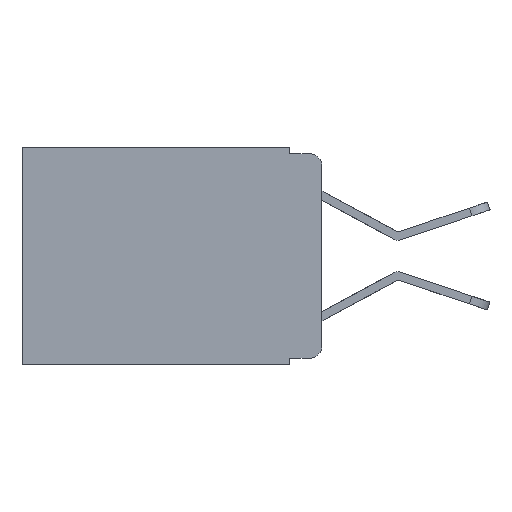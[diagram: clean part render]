
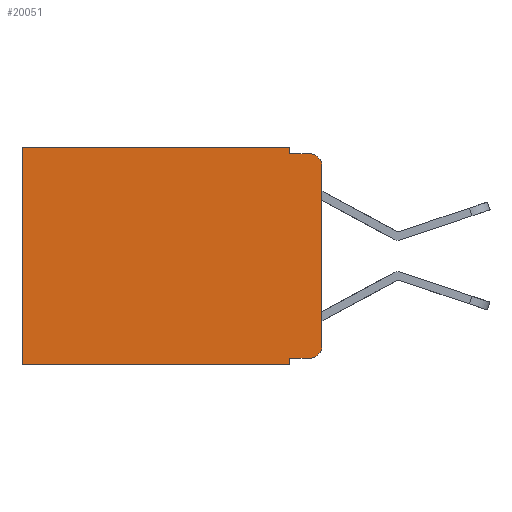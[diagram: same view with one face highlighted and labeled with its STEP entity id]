
A CAD part, left-side view. The second image highlights one B-rep face of the part: STEP entity #20051.
In plain terms, the highlighted planar face has unit normal (-1, 0, 0).
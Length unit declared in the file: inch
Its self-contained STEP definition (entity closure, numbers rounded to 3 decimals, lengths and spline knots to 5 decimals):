
#36 = EDGE_CURVE ( 'NONE', #19604, #1317, #16578, .T. ) ;
#1054 = ORIENTED_EDGE ( 'NONE', *, *, #10838, .F. ) ;
#1122 = DIRECTION ( 'NONE',  ( 0., -1., 0. ) ) ;
#1317 = VERTEX_POINT ( 'NONE', #21153 ) ;
#1393 = DIRECTION ( 'NONE',  ( 0., -1., 0. ) ) ;
#1402 = CARTESIAN_POINT ( 'NONE',  ( 0.298, 0.051, 0. ) ) ;
#1448 = EDGE_CURVE ( 'NONE', #19604, #22736, #23890, .T. ) ;
#1481 = CARTESIAN_POINT ( 'NONE',  ( 0.298, 0., -0.313 ) ) ;
#1501 = LINE ( 'NONE', #11058, #10415 ) ;
#1670 = DIRECTION ( 'NONE',  ( 0., 0., -1. ) ) ;
#1957 = CARTESIAN_POINT ( 'NONE',  ( 0.298, 0.051, -0.01 ) ) ;
#2050 = CARTESIAN_POINT ( 'NONE',  ( 0.298, 0.02, -0.313 ) ) ;
#2100 = AXIS2_PLACEMENT_3D ( 'NONE', #2050, #15978, #4168 ) ;
#2465 = LINE ( 'NONE', #7509, #22039 ) ;
#2858 = EDGE_CURVE ( 'NONE', #3120, #16821, #24452, .T. ) ;
#3104 = CARTESIAN_POINT ( 'NONE',  ( 0.298, 0.02, -0.01 ) ) ;
#3120 = VERTEX_POINT ( 'NONE', #21539 ) ;
#3197 = VERTEX_POINT ( 'NONE', #3104 ) ;
#3239 = CARTESIAN_POINT ( 'NONE',  ( 0.298, 0.051, 0. ) ) ;
#3483 = DIRECTION ( 'NONE',  ( 0., 0., -1. ) ) ;
#3519 = DIRECTION ( 'NONE',  ( -1., 0., 0. ) ) ;
#3686 = CARTESIAN_POINT ( 'NONE',  ( 0.298, 0., 0. ) ) ;
#4168 = DIRECTION ( 'NONE',  ( 0., 0., -1. ) ) ;
#4253 = EDGE_CURVE ( 'NONE', #15411, #4254, #9484, .T. ) ;
#4254 = VERTEX_POINT ( 'NONE', #1957 ) ;
#4309 = VECTOR ( 'NONE', #1393, 39.37008 ) ;
#4454 = EDGE_CURVE ( 'NONE', #15411, #3120, #1501, .T. ) ;
#6975 = EDGE_CURVE ( 'NONE', #4254, #3197, #14226, .T. ) ;
#7190 = ORIENTED_EDGE ( 'NONE', *, *, #1448, .F. ) ;
#7318 = VECTOR ( 'NONE', #12102, 39.37008 ) ;
#7509 = CARTESIAN_POINT ( 'NONE',  ( 0.298, 0., 0. ) ) ;
#8039 = CIRCLE ( 'NONE', #16832, 0.02 ) ;
#8131 = CARTESIAN_POINT ( 'NONE',  ( 0.298, 0., -0.343 ) ) ;
#8317 = EDGE_CURVE ( 'NONE', #8796, #3197, #8039, .T. ) ;
#8596 = VECTOR ( 'NONE', #13109, 39.37008 ) ;
#8783 = DIRECTION ( 'NONE',  ( 0., 0., -1. ) ) ;
#8796 = VERTEX_POINT ( 'NONE', #20344 ) ;
#9484 = LINE ( 'NONE', #24130, #24720 ) ;
#10415 = VECTOR ( 'NONE', #10828, 39.37008 ) ;
#10578 = CARTESIAN_POINT ( 'NONE',  ( 0.298, 0.473, 0. ) ) ;
#10595 = ORIENTED_EDGE ( 'NONE', *, *, #4253, .F. ) ;
#10678 = AXIS2_PLACEMENT_3D ( 'NONE', #3686, #13695, #1670 ) ;
#10828 = DIRECTION ( 'NONE',  ( 0., 1., 0. ) ) ;
#10838 = EDGE_CURVE ( 'NONE', #22736, #16821, #12561, .T. ) ;
#10939 = FACE_OUTER_BOUND ( 'NONE', #23181, .T. ) ;
#11058 = CARTESIAN_POINT ( 'NONE',  ( 0.298, 0., 0. ) ) ;
#11213 = ORIENTED_EDGE ( 'NONE', *, *, #4454, .T. ) ;
#11319 = EDGE_CURVE ( 'NONE', #8796, #13241, #2465, .T. ) ;
#11441 = VECTOR ( 'NONE', #1122, 39.37008 ) ;
#12102 = DIRECTION ( 'NONE',  ( 0., 1., 0. ) ) ;
#12432 = ORIENTED_EDGE ( 'NONE', *, *, #36, .T. ) ;
#12561 = LINE ( 'NONE', #8131, #7318 ) ;
#13080 = ORIENTED_EDGE ( 'NONE', *, *, #24193, .T. ) ;
#13109 = DIRECTION ( 'NONE',  ( 0., 0., -1. ) ) ;
#13241 = VERTEX_POINT ( 'NONE', #1481 ) ;
#13424 = CARTESIAN_POINT ( 'NONE',  ( 0.298, 0.051, -0.01 ) ) ;
#13695 = DIRECTION ( 'NONE',  ( 1., 0., 0. ) ) ;
#13886 = CARTESIAN_POINT ( 'NONE',  ( 0.298, 0.473, -0.343 ) ) ;
#13921 = ORIENTED_EDGE ( 'NONE', *, *, #11319, .F. ) ;
#14226 = LINE ( 'NONE', #13424, #4309 ) ;
#14827 = CARTESIAN_POINT ( 'NONE',  ( 0.298, 0.051, -0.343 ) ) ;
#15410 = CARTESIAN_POINT ( 'NONE',  ( 0.298, 0.02, -0.03 ) ) ;
#15411 = VERTEX_POINT ( 'NONE', #3239 ) ;
#15978 = DIRECTION ( 'NONE',  ( -1., 0., 0. ) ) ;
#16348 = ORIENTED_EDGE ( 'NONE', *, *, #2858, .T. ) ;
#16578 = LINE ( 'NONE', #19756, #11441 ) ;
#16821 = VERTEX_POINT ( 'NONE', #13886 ) ;
#16832 = AXIS2_PLACEMENT_3D ( 'NONE', #15410, #3519, #17340 ) ;
#17029 = CIRCLE ( 'NONE', #2100, 0.02 ) ;
#17340 = DIRECTION ( 'NONE',  ( 0., 0., -1. ) ) ;
#19479 = VECTOR ( 'NONE', #8783, 39.37008 ) ;
#19604 = VERTEX_POINT ( 'NONE', #21863 ) ;
#19756 = CARTESIAN_POINT ( 'NONE',  ( 0.298, 0.051, -0.333 ) ) ;
#20051 = ADVANCED_FACE ( 'NONE', ( #10939 ), #25041, .F. ) ;
#20344 = CARTESIAN_POINT ( 'NONE',  ( 0.298, 0., -0.03 ) ) ;
#21153 = CARTESIAN_POINT ( 'NONE',  ( 0.298, 0.02, -0.333 ) ) ;
#21539 = CARTESIAN_POINT ( 'NONE',  ( 0.298, 0.473, 0. ) ) ;
#21858 = DIRECTION ( 'NONE',  ( 0., 0., -1. ) ) ;
#21863 = CARTESIAN_POINT ( 'NONE',  ( 0.298, 0.051, -0.333 ) ) ;
#22039 = VECTOR ( 'NONE', #3483, 39.37008 ) ;
#22736 = VERTEX_POINT ( 'NONE', #14827 ) ;
#23181 = EDGE_LOOP ( 'NONE', ( #13921, #24594, #25186, #10595, #11213, #16348, #1054, #7190, #12432, #13080 ) ) ;
#23890 = LINE ( 'NONE', #1402, #8596 ) ;
#24130 = CARTESIAN_POINT ( 'NONE',  ( 0.298, 0.051, 0. ) ) ;
#24193 = EDGE_CURVE ( 'NONE', #1317, #13241, #17029, .T. ) ;
#24452 = LINE ( 'NONE', #10578, #19479 ) ;
#24594 = ORIENTED_EDGE ( 'NONE', *, *, #8317, .T. ) ;
#24720 = VECTOR ( 'NONE', #21858, 39.37008 ) ;
#25041 = PLANE ( 'NONE',  #10678 ) ;
#25186 = ORIENTED_EDGE ( 'NONE', *, *, #6975, .F. ) ;
